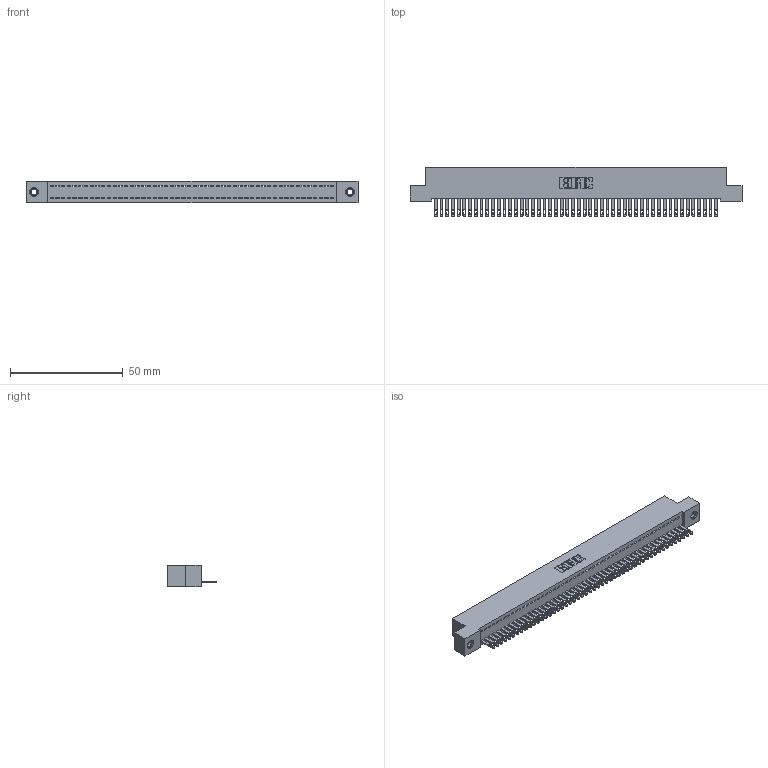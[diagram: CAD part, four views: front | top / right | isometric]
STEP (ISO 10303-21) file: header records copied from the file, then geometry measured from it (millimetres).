
FILE_DESCRIPTION (( 'STEP AP203' ), '1' );
FILE_NAME ('892-050-500-107.STEP', '2020-09-21T17:47:14', ( '' ), ( '' ), 'SwSTEP 2.0', 'SolidWorks 2020', '' );
FILE_SCHEMA (( 'CONFIG_CONTROL_DESIGN' ));
Length unit declared in the file: inch
Products named in the file (4): 892-050-500-107; 842 Part_TI; 345-292-001_345-293-100; 345-250-001_345-250-005-103
Assembly tree (53 placements, depth 2):
  892-050-500-107
    842 Part_TI
    345-292-001_345-293-100  x50
    345-250-001_345-250-005-103  x2
Bounding box: 147.32 x 21.85 x 9.4 mm (x, y, z)
Volume: 12964.7 mm3; surface area: 19318.1 mm2
Topology: 53 solids, 53 shells, 2870 faces, 8835 edges, 5882 vertices
Faces by surface type: plane 1898, cylinder 956, cone 12, torus 4
Entity records: 30516 total; most frequent: CARTESIAN_POINT 5243, ORIENTED_EDGE 5222, DIRECTION 4441, EDGE_CURVE 2611, LINE 2459, VECTOR 2459, VERTEX_POINT 1736, AXIS2_PLACEMENT_3D 991
